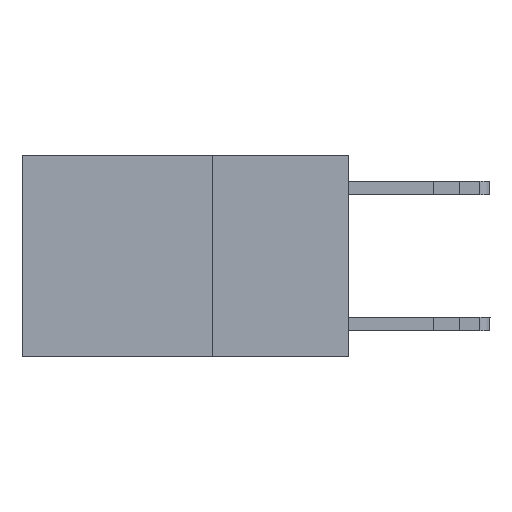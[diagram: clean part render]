
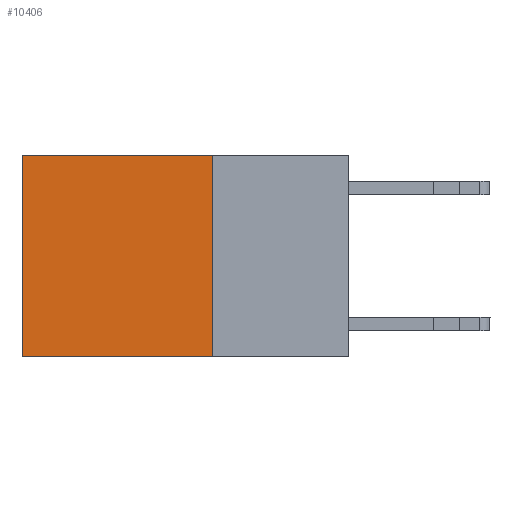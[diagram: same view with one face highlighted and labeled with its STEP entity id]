
A CAD part, left-side view. The second image highlights one B-rep face of the part: STEP entity #10406.
In plain terms, the highlighted planar face has unit normal (-1, 0, 0).
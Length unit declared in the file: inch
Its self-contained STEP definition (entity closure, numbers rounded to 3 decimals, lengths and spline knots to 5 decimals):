
#1446 = ORIENTED_EDGE ( 'NONE', *, *, #2064, .F. ) ;
#2064 = EDGE_CURVE ( 'NONE', #5445, #12859, #7056, .T. ) ;
#2204 = EDGE_LOOP ( 'NONE', ( #16221, #1446, #19512, #22312 ) ) ;
#3483 = DIRECTION ( 'NONE',  ( 0., 1., 0. ) ) ;
#3718 = CARTESIAN_POINT ( 'NONE',  ( 0.2625, 0.25, -0.37 ) ) ;
#3858 = VECTOR ( 'NONE', #8192, 39.37008 ) ;
#4140 = LINE ( 'NONE', #8582, #3858 ) ;
#5445 = VERTEX_POINT ( 'NONE', #8739 ) ;
#5896 = EDGE_CURVE ( 'NONE', #15038, #5445, #4140, .T. ) ;
#6407 = DIRECTION ( 'NONE',  ( 0., 0., -1. ) ) ;
#6582 = PLANE ( 'NONE',  #21393 ) ;
#6635 = CARTESIAN_POINT ( 'NONE',  ( 0.2625, 0.25, 0. ) ) ;
#6905 = VECTOR ( 'NONE', #3483, 39.37008 ) ;
#7056 = LINE ( 'NONE', #3718, #6905 ) ;
#7136 = DIRECTION ( 'NONE',  ( 1., 0., 0. ) ) ;
#7906 = VECTOR ( 'NONE', #18660, 39.37008 ) ;
#8192 = DIRECTION ( 'NONE',  ( 0., 0., -1. ) ) ;
#8582 = CARTESIAN_POINT ( 'NONE',  ( 0.2625, 0.25, 0. ) ) ;
#8739 = CARTESIAN_POINT ( 'NONE',  ( 0.2625, 0.25, -0.37 ) ) ;
#9238 = EDGE_CURVE ( 'NONE', #15038, #11180, #16346, .T. ) ;
#9487 = VECTOR ( 'NONE', #16287, 39.37008 ) ;
#9571 = LINE ( 'NONE', #21432, #9487 ) ;
#10406 = ADVANCED_FACE ( 'NONE', ( #16891 ), #6582, .F. ) ;
#10489 = CARTESIAN_POINT ( 'NONE',  ( 0.2625, 0.6, -0.37 ) ) ;
#11180 = VERTEX_POINT ( 'NONE', #18102 ) ;
#12859 = VERTEX_POINT ( 'NONE', #10489 ) ;
#15038 = VERTEX_POINT ( 'NONE', #15240 ) ;
#15240 = CARTESIAN_POINT ( 'NONE',  ( 0.2625, 0.25, 0. ) ) ;
#16221 = ORIENTED_EDGE ( 'NONE', *, *, #22380, .T. ) ;
#16287 = DIRECTION ( 'NONE',  ( 0., 0., -1. ) ) ;
#16346 = LINE ( 'NONE', #21802, #7906 ) ;
#16891 = FACE_OUTER_BOUND ( 'NONE', #2204, .T. ) ;
#18102 = CARTESIAN_POINT ( 'NONE',  ( 0.2625, 0.6, 0. ) ) ;
#18660 = DIRECTION ( 'NONE',  ( 0., 1., 0. ) ) ;
#19512 = ORIENTED_EDGE ( 'NONE', *, *, #5896, .F. ) ;
#21393 = AXIS2_PLACEMENT_3D ( 'NONE', #6635, #7136, #6407 ) ;
#21432 = CARTESIAN_POINT ( 'NONE',  ( 0.2625, 0.6, 0. ) ) ;
#21802 = CARTESIAN_POINT ( 'NONE',  ( 0.2625, 0.25, 0. ) ) ;
#22312 = ORIENTED_EDGE ( 'NONE', *, *, #9238, .T. ) ;
#22380 = EDGE_CURVE ( 'NONE', #11180, #12859, #9571, .T. ) ;
